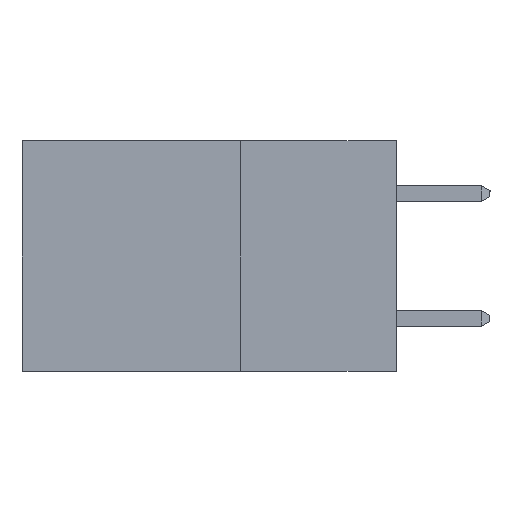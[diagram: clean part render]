
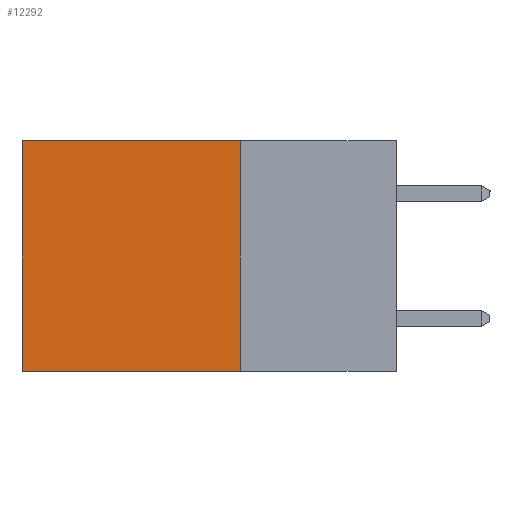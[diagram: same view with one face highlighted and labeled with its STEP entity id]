
A CAD part, left-side view. The second image highlights one B-rep face of the part: STEP entity #12292.
In plain terms, the highlighted planar face has unit normal (-1, 0, 0).
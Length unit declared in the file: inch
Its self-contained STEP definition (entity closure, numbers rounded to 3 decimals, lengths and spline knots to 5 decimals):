
#575 = EDGE_CURVE ( 'NONE', #4984, #12111, #659, .T. ) ;
#659 = LINE ( 'NONE', #9064, #1966 ) ;
#1578 = ORIENTED_EDGE ( 'NONE', *, *, #8446, .F. ) ;
#1659 = ORIENTED_EDGE ( 'NONE', *, *, #13615, .T. ) ;
#1966 = VECTOR ( 'NONE', #8005, 39.37008 ) ;
#2497 = VERTEX_POINT ( 'NONE', #4603 ) ;
#2672 = ORIENTED_EDGE ( 'NONE', *, *, #575, .T. ) ;
#2935 = FACE_OUTER_BOUND ( 'NONE', #13469, .T. ) ;
#3490 = LINE ( 'NONE', #4592, #8236 ) ;
#4491 = CARTESIAN_POINT ( 'NONE',  ( 0.2615, 0.25, -0.37 ) ) ;
#4514 = DIRECTION ( 'NONE',  ( 0., 1., 0. ) ) ;
#4592 = CARTESIAN_POINT ( 'NONE',  ( 0.2615, 0.25, 0. ) ) ;
#4603 = CARTESIAN_POINT ( 'NONE',  ( 0.2615, 0.25, -0.37 ) ) ;
#4984 = VERTEX_POINT ( 'NONE', #12736 ) ;
#5490 = VECTOR ( 'NONE', #10837, 39.37008 ) ;
#5659 = CARTESIAN_POINT ( 'NONE',  ( 0.2615, 0.25, -0.37 ) ) ;
#6375 = DIRECTION ( 'NONE',  ( 1., 0., 0. ) ) ;
#6919 = CARTESIAN_POINT ( 'NONE',  ( 0.2615, 0.6, -0.37 ) ) ;
#6929 = EDGE_CURVE ( 'NONE', #2497, #12111, #7301, .T. ) ;
#7301 = LINE ( 'NONE', #4491, #5490 ) ;
#7573 = VECTOR ( 'NONE', #14386, 39.37008 ) ;
#7812 = PLANE ( 'NONE',  #14682 ) ;
#8005 = DIRECTION ( 'NONE',  ( 0., 0., -1. ) ) ;
#8236 = VECTOR ( 'NONE', #4514, 39.37008 ) ;
#8446 = EDGE_CURVE ( 'NONE', #10340, #2497, #9438, .T. ) ;
#8957 = CARTESIAN_POINT ( 'NONE',  ( 0.2615, 0.25, -0.37 ) ) ;
#9064 = CARTESIAN_POINT ( 'NONE',  ( 0.2615, 0.6, -0.37 ) ) ;
#9438 = LINE ( 'NONE', #5659, #7573 ) ;
#9718 = ORIENTED_EDGE ( 'NONE', *, *, #6929, .F. ) ;
#10340 = VERTEX_POINT ( 'NONE', #11824 ) ;
#10837 = DIRECTION ( 'NONE',  ( 0., 1., 0. ) ) ;
#11824 = CARTESIAN_POINT ( 'NONE',  ( 0.2615, 0.25, 0. ) ) ;
#12111 = VERTEX_POINT ( 'NONE', #6919 ) ;
#12292 = ADVANCED_FACE ( 'NONE', ( #2935 ), #7812, .F. ) ;
#12472 = DIRECTION ( 'NONE',  ( 0., 0., -1. ) ) ;
#12736 = CARTESIAN_POINT ( 'NONE',  ( 0.2615, 0.6, 0. ) ) ;
#13469 = EDGE_LOOP ( 'NONE', ( #2672, #9718, #1578, #1659 ) ) ;
#13615 = EDGE_CURVE ( 'NONE', #10340, #4984, #3490, .T. ) ;
#14386 = DIRECTION ( 'NONE',  ( 0., 0., -1. ) ) ;
#14682 = AXIS2_PLACEMENT_3D ( 'NONE', #8957, #6375, #12472 ) ;
